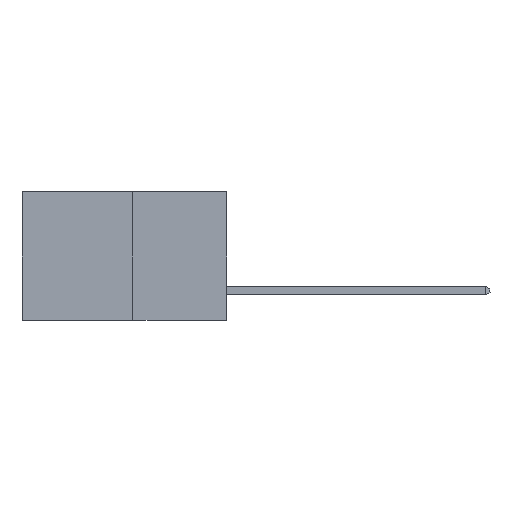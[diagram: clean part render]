
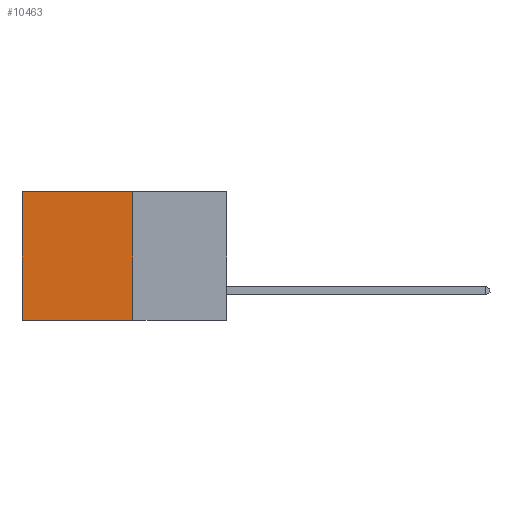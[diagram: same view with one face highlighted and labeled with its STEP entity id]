
A CAD part, left-side view. The second image highlights one B-rep face of the part: STEP entity #10463.
In plain terms, the highlighted planar face has unit normal (-1, 0, 0).
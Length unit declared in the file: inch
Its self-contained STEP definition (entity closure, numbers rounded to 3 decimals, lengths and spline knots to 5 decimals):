
#716 = VERTEX_POINT ( 'NONE', #6292 ) ;
#999 = EDGE_CURVE ( 'NONE', #7806, #716, #2433, .T. ) ;
#1135 = FACE_OUTER_BOUND ( 'NONE', #10691, .T. ) ;
#1176 = EDGE_CURVE ( 'NONE', #3743, #11436, #9761, .T. ) ;
#1420 = AXIS2_PLACEMENT_3D ( 'NONE', #3077, #11134, #5839 ) ;
#1536 = DIRECTION ( 'NONE',  ( 0., 0., -1. ) ) ;
#1663 = CARTESIAN_POINT ( 'NONE',  ( 0.277, 0.27, 0. ) ) ;
#2433 = LINE ( 'NONE', #3591, #7273 ) ;
#2652 = LINE ( 'NONE', #1663, #6649 ) ;
#2860 = CARTESIAN_POINT ( 'NONE',  ( 0.277, 0.27, -0.37 ) ) ;
#3076 = DIRECTION ( 'NONE',  ( 0., 0., -1. ) ) ;
#3077 = CARTESIAN_POINT ( 'NONE',  ( 0.277, 0.27, -0.37 ) ) ;
#3591 = CARTESIAN_POINT ( 'NONE',  ( 0.277, 0.59, -0.37 ) ) ;
#3743 = VERTEX_POINT ( 'NONE', #11579 ) ;
#4081 = EDGE_CURVE ( 'NONE', #11436, #716, #11633, .T. ) ;
#4931 = PLANE ( 'NONE',  #1420 ) ;
#5366 = ORIENTED_EDGE ( 'NONE', *, *, #1176, .F. ) ;
#5839 = DIRECTION ( 'NONE',  ( 0., 0., -1. ) ) ;
#6048 = CARTESIAN_POINT ( 'NONE',  ( 0.277, 0.59, 0. ) ) ;
#6292 = CARTESIAN_POINT ( 'NONE',  ( 0.277, 0.59, -0.37 ) ) ;
#6649 = VECTOR ( 'NONE', #8882, 39.37008 ) ;
#7273 = VECTOR ( 'NONE', #3076, 39.37008 ) ;
#7411 = VECTOR ( 'NONE', #1536, 39.37008 ) ;
#7461 = ORIENTED_EDGE ( 'NONE', *, *, #999, .T. ) ;
#7806 = VERTEX_POINT ( 'NONE', #6048 ) ;
#8882 = DIRECTION ( 'NONE',  ( 0., 1., 0. ) ) ;
#9286 = DIRECTION ( 'NONE',  ( 0., 1., 0. ) ) ;
#9300 = CARTESIAN_POINT ( 'NONE',  ( 0.277, 0.27, -0.37 ) ) ;
#9694 = CARTESIAN_POINT ( 'NONE',  ( 0.277, 0.27, -0.37 ) ) ;
#9761 = LINE ( 'NONE', #9694, #7411 ) ;
#9808 = ORIENTED_EDGE ( 'NONE', *, *, #4081, .F. ) ;
#10077 = ORIENTED_EDGE ( 'NONE', *, *, #10739, .T. ) ;
#10114 = VECTOR ( 'NONE', #9286, 39.37008 ) ;
#10463 = ADVANCED_FACE ( 'NONE', ( #1135 ), #4931, .F. ) ;
#10691 = EDGE_LOOP ( 'NONE', ( #7461, #9808, #5366, #10077 ) ) ;
#10739 = EDGE_CURVE ( 'NONE', #3743, #7806, #2652, .T. ) ;
#11134 = DIRECTION ( 'NONE',  ( 1., 0., 0. ) ) ;
#11436 = VERTEX_POINT ( 'NONE', #2860 ) ;
#11579 = CARTESIAN_POINT ( 'NONE',  ( 0.277, 0.27, 0. ) ) ;
#11633 = LINE ( 'NONE', #9300, #10114 ) ;
